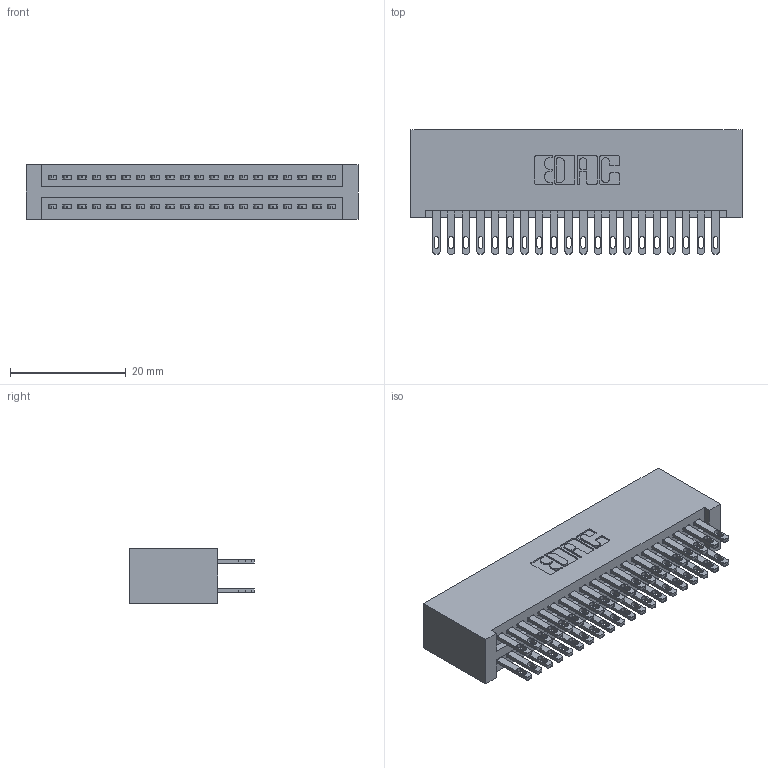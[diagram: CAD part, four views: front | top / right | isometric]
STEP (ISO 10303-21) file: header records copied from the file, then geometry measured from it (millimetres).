
FILE_DESCRIPTION (( 'STEP AP203' ), '1' );
FILE_NAME ('345-040-500-201.STEP', '2019-10-28T16:27:39', ( '' ), ( '' ), 'SwSTEP 2.0', 'SolidWorks 2016', '' );
FILE_SCHEMA (( 'CONFIG_CONTROL_DESIGN' ));
Length unit declared in the file: inch
Products named in the file (3): 345-292-001_345-293-100; 345 Part_No Mounting Lugs; 345-040-500-201
Assembly tree (41 placements, depth 2):
  345-040-500-201
    345 Part_No Mounting Lugs
    345-292-001_345-293-100  x40
Bounding box: 57.4 x 21.51 x 9.4 mm (x, y, z)
Volume: 6110.2 mm3; surface area: 9317.1 mm2
Topology: 41 solids, 41 shells, 1958 faces, 5957 edges, 3970 vertices
Faces by surface type: plane 1156, cylinder 802
Entity records: 18307 total; most frequent: CARTESIAN_POINT 3088, ORIENTED_EDGE 3022, DIRECTION 2747, EDGE_CURVE 1511, LINE 1303, VECTOR 1303, VERTEX_POINT 1006, AXIS2_PLACEMENT_3D 722
